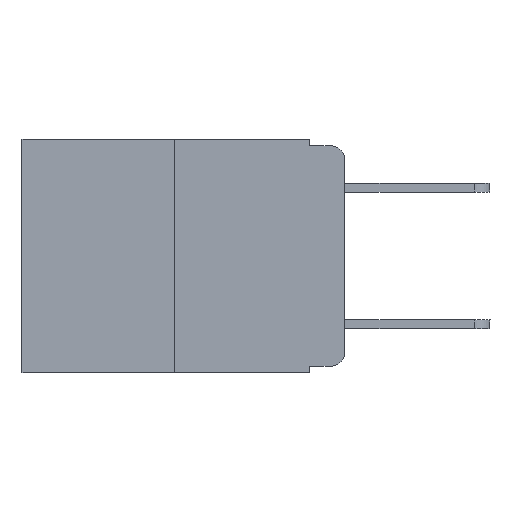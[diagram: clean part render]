
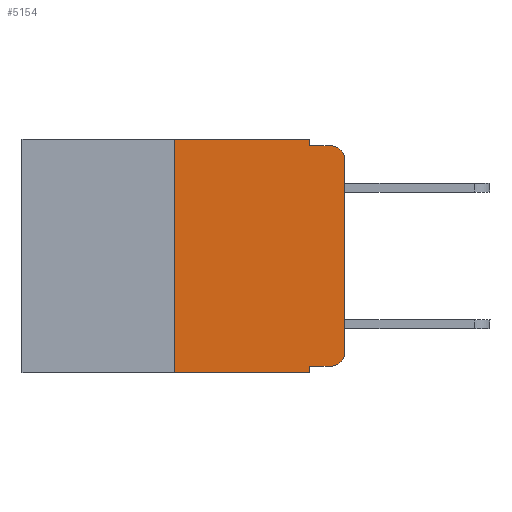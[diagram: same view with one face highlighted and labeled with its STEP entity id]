
A CAD part, left-side view. The second image highlights one B-rep face of the part: STEP entity #5154.
In plain terms, the highlighted planar face has unit normal (-1, 0, 0).
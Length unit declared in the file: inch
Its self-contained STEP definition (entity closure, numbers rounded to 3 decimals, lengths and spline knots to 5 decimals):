
#127 = VERTEX_POINT ( 'NONE', #888 ) ;
#270 = LINE ( 'NONE', #11545, #7542 ) ;
#421 = VERTEX_POINT ( 'NONE', #10161 ) ;
#775 = CARTESIAN_POINT ( 'NONE',  ( 0., 0.02, -0.01 ) ) ;
#790 = EDGE_CURVE ( 'NONE', #16061, #15442, #6116, .T. ) ;
#826 = DIRECTION ( 'NONE',  ( 0., -1., 0. ) ) ;
#888 = CARTESIAN_POINT ( 'NONE',  ( 0., 0.25, -0.343 ) ) ;
#1147 = ORIENTED_EDGE ( 'NONE', *, *, #790, .F. ) ;
#1188 = CARTESIAN_POINT ( 'NONE',  ( 0., 0.051, 0. ) ) ;
#1253 = DIRECTION ( 'NONE',  ( -1., 0., 0. ) ) ;
#1428 = DIRECTION ( 'NONE',  ( 0., 0., -1. ) ) ;
#1520 = VERTEX_POINT ( 'NONE', #775 ) ;
#1768 = VECTOR ( 'NONE', #1990, 39.37008 ) ;
#1990 = DIRECTION ( 'NONE',  ( 0., 0., 1. ) ) ;
#2009 = VECTOR ( 'NONE', #826, 39.37008 ) ;
#2287 = CARTESIAN_POINT ( 'NONE',  ( 0., 0.051, -0.01 ) ) ;
#2441 = DIRECTION ( 'NONE',  ( 0., -1., 0. ) ) ;
#2617 = CARTESIAN_POINT ( 'NONE',  ( 0., 0.473, -0.343 ) ) ;
#2673 = VECTOR ( 'NONE', #14541, 39.37008 ) ;
#3246 = CIRCLE ( 'NONE', #15467, 0.02 ) ;
#3466 = EDGE_CURVE ( 'NONE', #8566, #421, #12864, .T. ) ;
#3755 = ORIENTED_EDGE ( 'NONE', *, *, #13048, .T. ) ;
#4340 = CARTESIAN_POINT ( 'NONE',  ( 0., 0., -0.03 ) ) ;
#4617 = VERTEX_POINT ( 'NONE', #4340 ) ;
#5154 = ADVANCED_FACE ( 'NONE', ( #5842 ), #21081, .F. ) ;
#5223 = DIRECTION ( 'NONE',  ( 0., 0., 1. ) ) ;
#5345 = CARTESIAN_POINT ( 'NONE',  ( 0., 0.25, 0. ) ) ;
#5840 = CARTESIAN_POINT ( 'NONE',  ( 0., 0.051, -0.343 ) ) ;
#5842 = FACE_OUTER_BOUND ( 'NONE', #16361, .T. ) ;
#6116 = LINE ( 'NONE', #1188, #2673 ) ;
#6356 = VECTOR ( 'NONE', #17732, 39.37008 ) ;
#6697 = EDGE_CURVE ( 'NONE', #127, #17262, #10513, .T. ) ;
#7354 = CARTESIAN_POINT ( 'NONE',  ( 0., 0.051, 0. ) ) ;
#7403 = EDGE_CURVE ( 'NONE', #8566, #8377, #11035, .T. ) ;
#7542 = VECTOR ( 'NONE', #5223, 39.37008 ) ;
#7591 = ORIENTED_EDGE ( 'NONE', *, *, #6697, .F. ) ;
#7929 = DIRECTION ( 'NONE',  ( 0., 0., -1. ) ) ;
#8223 = ORIENTED_EDGE ( 'NONE', *, *, #16245, .T. ) ;
#8331 = ORIENTED_EDGE ( 'NONE', *, *, #3466, .T. ) ;
#8377 = VERTEX_POINT ( 'NONE', #5840 ) ;
#8566 = VERTEX_POINT ( 'NONE', #21293 ) ;
#9116 = ORIENTED_EDGE ( 'NONE', *, *, #7403, .F. ) ;
#9962 = EDGE_CURVE ( 'NONE', #421, #18238, #3246, .T. ) ;
#10036 = AXIS2_PLACEMENT_3D ( 'NONE', #13155, #11727, #18323 ) ;
#10073 = VECTOR ( 'NONE', #12915, 39.37008 ) ;
#10161 = CARTESIAN_POINT ( 'NONE',  ( 0., 0.02, -0.333 ) ) ;
#10273 = EDGE_CURVE ( 'NONE', #15442, #1520, #15686, .T. ) ;
#10513 = LINE ( 'NONE', #16998, #1768 ) ;
#11035 = LINE ( 'NONE', #21145, #6356 ) ;
#11545 = CARTESIAN_POINT ( 'NONE',  ( 0., 0., 0. ) ) ;
#11727 = DIRECTION ( 'NONE',  ( -1., 0., 0. ) ) ;
#11814 = ORIENTED_EDGE ( 'NONE', *, *, #10273, .F. ) ;
#12470 = DIRECTION ( 'NONE',  ( 0., -1., 0. ) ) ;
#12864 = LINE ( 'NONE', #20902, #2009 ) ;
#12915 = DIRECTION ( 'NONE',  ( 0., -1., 0. ) ) ;
#13048 = EDGE_CURVE ( 'NONE', #18238, #4617, #270, .T. ) ;
#13155 = CARTESIAN_POINT ( 'NONE',  ( 0., 0.02, -0.03 ) ) ;
#13194 = CIRCLE ( 'NONE', #10036, 0.02 ) ;
#14016 = VECTOR ( 'NONE', #12470, 39.37008 ) ;
#14314 = CARTESIAN_POINT ( 'NONE',  ( 0., 0., -0.313 ) ) ;
#14541 = DIRECTION ( 'NONE',  ( 0., 0., -1. ) ) ;
#15442 = VERTEX_POINT ( 'NONE', #2287 ) ;
#15467 = AXIS2_PLACEMENT_3D ( 'NONE', #16260, #1253, #7929 ) ;
#15483 = VECTOR ( 'NONE', #2441, 39.37008 ) ;
#15683 = CARTESIAN_POINT ( 'NONE',  ( 0., 0.473, 0. ) ) ;
#15686 = LINE ( 'NONE', #17456, #15483 ) ;
#15775 = LINE ( 'NONE', #21279, #10073 ) ;
#16061 = VERTEX_POINT ( 'NONE', #7354 ) ;
#16180 = AXIS2_PLACEMENT_3D ( 'NONE', #15683, #21297, #1428 ) ;
#16245 = EDGE_CURVE ( 'NONE', #4617, #1520, #13194, .T. ) ;
#16260 = CARTESIAN_POINT ( 'NONE',  ( 0., 0.02, -0.313 ) ) ;
#16361 = EDGE_LOOP ( 'NONE', ( #3755, #8223, #11814, #1147, #19788, #7591, #19601, #9116, #8331, #18235 ) ) ;
#16998 = CARTESIAN_POINT ( 'NONE',  ( 0., 0.25, 0. ) ) ;
#17262 = VERTEX_POINT ( 'NONE', #5345 ) ;
#17456 = CARTESIAN_POINT ( 'NONE',  ( 0., 0.051, -0.01 ) ) ;
#17732 = DIRECTION ( 'NONE',  ( 0., 0., -1. ) ) ;
#17898 = EDGE_CURVE ( 'NONE', #17262, #16061, #15775, .T. ) ;
#18235 = ORIENTED_EDGE ( 'NONE', *, *, #9962, .T. ) ;
#18238 = VERTEX_POINT ( 'NONE', #14314 ) ;
#18323 = DIRECTION ( 'NONE',  ( 0., 0., -1. ) ) ;
#19601 = ORIENTED_EDGE ( 'NONE', *, *, #20554, .T. ) ;
#19788 = ORIENTED_EDGE ( 'NONE', *, *, #17898, .F. ) ;
#20554 = EDGE_CURVE ( 'NONE', #127, #8377, #21152, .T. ) ;
#20902 = CARTESIAN_POINT ( 'NONE',  ( 0., 0.051, -0.333 ) ) ;
#21081 = PLANE ( 'NONE',  #16180 ) ;
#21145 = CARTESIAN_POINT ( 'NONE',  ( 0., 0.051, 0. ) ) ;
#21152 = LINE ( 'NONE', #2617, #14016 ) ;
#21279 = CARTESIAN_POINT ( 'NONE',  ( 0., 0.473, 0. ) ) ;
#21293 = CARTESIAN_POINT ( 'NONE',  ( 0., 0.051, -0.333 ) ) ;
#21297 = DIRECTION ( 'NONE',  ( 1., 0., 0. ) ) ;
